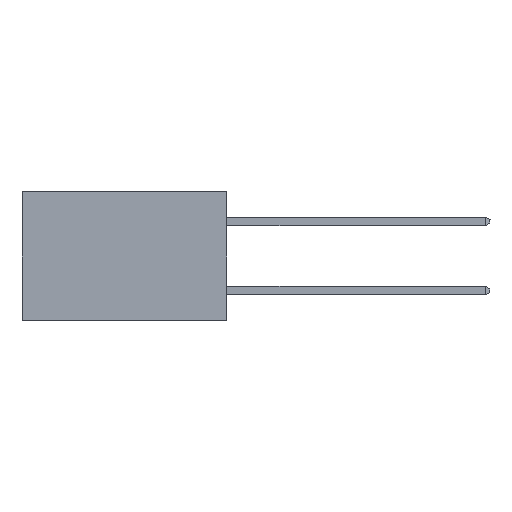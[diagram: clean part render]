
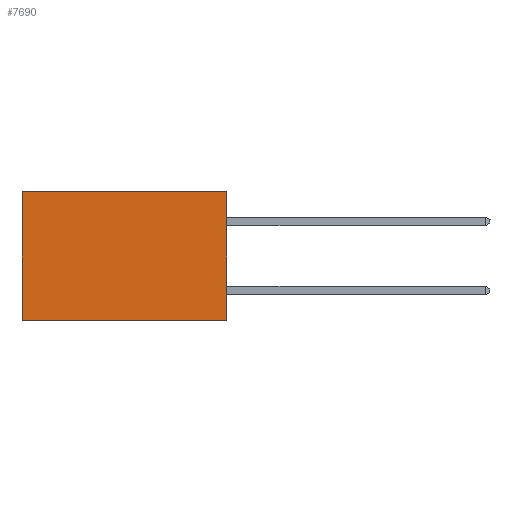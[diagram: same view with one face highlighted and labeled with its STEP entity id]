
A CAD part, left-side view. The second image highlights one B-rep face of the part: STEP entity #7690.
In plain terms, the highlighted planar face has unit normal (-1, 0, 0).
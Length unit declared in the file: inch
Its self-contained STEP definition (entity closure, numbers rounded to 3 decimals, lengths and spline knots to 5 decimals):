
#343 = DIRECTION ( 'NONE',  ( 1., 0., 0. ) ) ;
#814 = EDGE_CURVE ( 'NONE', #22624, #27823, #18531, .T. ) ;
#1886 = CARTESIAN_POINT ( 'NONE',  ( 0.277, 0.59, -0.37 ) ) ;
#2362 = CARTESIAN_POINT ( 'NONE',  ( 0.277, 0., -0.37 ) ) ;
#2445 = EDGE_CURVE ( 'NONE', #13110, #27823, #5875, .T. ) ;
#4211 = VECTOR ( 'NONE', #13379, 39.37008 ) ;
#5675 = AXIS2_PLACEMENT_3D ( 'NONE', #29676, #343, #19158 ) ;
#5875 = LINE ( 'NONE', #13411, #4211 ) ;
#6316 = FACE_OUTER_BOUND ( 'NONE', #22219, .T. ) ;
#6901 = LINE ( 'NONE', #9240, #14885 ) ;
#7690 = ADVANCED_FACE ( 'NONE', ( #6316 ), #26993, .F. ) ;
#8417 = EDGE_CURVE ( 'NONE', #18157, #22624, #25948, .T. ) ;
#9240 = CARTESIAN_POINT ( 'NONE',  ( 0.277, 0., -0.37 ) ) ;
#9957 = ORIENTED_EDGE ( 'NONE', *, *, #2445, .F. ) ;
#12661 = CARTESIAN_POINT ( 'NONE',  ( 0.277, 0.59, 0. ) ) ;
#13110 = VERTEX_POINT ( 'NONE', #2362 ) ;
#13379 = DIRECTION ( 'NONE',  ( 0., 1., 0. ) ) ;
#13411 = CARTESIAN_POINT ( 'NONE',  ( 0.277, 0., -0.37 ) ) ;
#13647 = ORIENTED_EDGE ( 'NONE', *, *, #814, .T. ) ;
#14209 = DIRECTION ( 'NONE',  ( 0., 1., 0. ) ) ;
#14885 = VECTOR ( 'NONE', #25221, 39.37008 ) ;
#16310 = ORIENTED_EDGE ( 'NONE', *, *, #8417, .T. ) ;
#18157 = VERTEX_POINT ( 'NONE', #24680 ) ;
#18325 = EDGE_CURVE ( 'NONE', #18157, #13110, #6901, .T. ) ;
#18531 = LINE ( 'NONE', #24393, #33522 ) ;
#18933 = VECTOR ( 'NONE', #14209, 39.37008 ) ;
#19158 = DIRECTION ( 'NONE',  ( 0., 0., -1. ) ) ;
#22219 = EDGE_LOOP ( 'NONE', ( #13647, #9957, #26069, #16310 ) ) ;
#22624 = VERTEX_POINT ( 'NONE', #12661 ) ;
#24393 = CARTESIAN_POINT ( 'NONE',  ( 0.277, 0.59, -0.37 ) ) ;
#24456 = DIRECTION ( 'NONE',  ( 0., 0., -1. ) ) ;
#24680 = CARTESIAN_POINT ( 'NONE',  ( 0.277, 0., 0. ) ) ;
#25221 = DIRECTION ( 'NONE',  ( 0., 0., -1. ) ) ;
#25948 = LINE ( 'NONE', #27415, #18933 ) ;
#26069 = ORIENTED_EDGE ( 'NONE', *, *, #18325, .F. ) ;
#26993 = PLANE ( 'NONE',  #5675 ) ;
#27415 = CARTESIAN_POINT ( 'NONE',  ( 0.277, 0., 0. ) ) ;
#27823 = VERTEX_POINT ( 'NONE', #1886 ) ;
#29676 = CARTESIAN_POINT ( 'NONE',  ( 0.277, 0., -0.37 ) ) ;
#33522 = VECTOR ( 'NONE', #24456, 39.37008 ) ;
